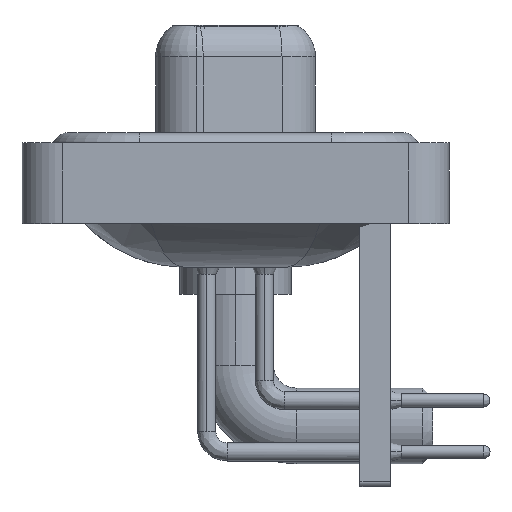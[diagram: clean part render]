
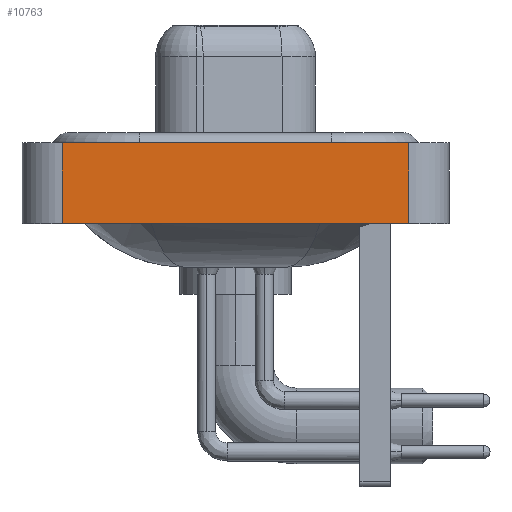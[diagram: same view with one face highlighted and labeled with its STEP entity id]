
A CAD part, left-side view. The second image highlights one B-rep face of the part: STEP entity #10763.
In plain terms, the highlighted planar face has unit normal (-1, 0, 0).
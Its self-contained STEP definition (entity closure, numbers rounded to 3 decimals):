
#282 = CARTESIAN_POINT ( 'NONE',  ( -7.25, -8.55, -3.6 ) ) ;
#705 = VERTEX_POINT ( 'NONE', #17189 ) ;
#1591 = EDGE_CURVE ( 'NONE', #705, #3271, #16674, .T. ) ;
#1983 = EDGE_CURVE ( 'NONE', #16184, #3271, #9719, .T. ) ;
#2035 = VECTOR ( 'NONE', #11398, 1000. ) ;
#2702 = VECTOR ( 'NONE', #7705, 1000. ) ;
#2917 = CARTESIAN_POINT ( 'NONE',  ( -7.25, -8.55, 0.4 ) ) ;
#3153 = ORIENTED_EDGE ( 'NONE', *, *, #8370, .F. ) ;
#3271 = VERTEX_POINT ( 'NONE', #2917 ) ;
#3435 = CARTESIAN_POINT ( 'NONE',  ( -7.25, 8.55, -3.6 ) ) ;
#3968 = DIRECTION ( 'NONE',  ( 0., -1., 0. ) ) ;
#4445 = LINE ( 'NONE', #12413, #2702 ) ;
#5034 = ORIENTED_EDGE ( 'NONE', *, *, #1983, .T. ) ;
#5622 = LINE ( 'NONE', #20192, #10661 ) ;
#5769 = AXIS2_PLACEMENT_3D ( 'NONE', #12751, #14438, #7633 ) ;
#5783 = ORIENTED_EDGE ( 'NONE', *, *, #9924, .T. ) ;
#5931 = DIRECTION ( 'NONE',  ( 0., 0., 1. ) ) ;
#7025 = CARTESIAN_POINT ( 'NONE',  ( -7.25, -8.55, 0.4 ) ) ;
#7633 = DIRECTION ( 'NONE',  ( 0., 0., 1. ) ) ;
#7705 = DIRECTION ( 'NONE',  ( 0., -1., 0. ) ) ;
#8370 = EDGE_CURVE ( 'NONE', #14598, #705, #5622, .T. ) ;
#9719 = LINE ( 'NONE', #282, #2035 ) ;
#9924 = EDGE_CURVE ( 'NONE', #14598, #16184, #4445, .T. ) ;
#10661 = VECTOR ( 'NONE', #5931, 1000. ) ;
#10667 = FACE_OUTER_BOUND ( 'NONE', #15027, .T. ) ;
#10763 = ADVANCED_FACE ( 'NONE', ( #10667 ), #17382, .T. ) ;
#11398 = DIRECTION ( 'NONE',  ( 0., 0., 1. ) ) ;
#12413 = CARTESIAN_POINT ( 'NONE',  ( -7.25, -8.55, -3.6 ) ) ;
#12601 = ORIENTED_EDGE ( 'NONE', *, *, #1591, .F. ) ;
#12751 = CARTESIAN_POINT ( 'NONE',  ( -7.25, -8.55, -3.6 ) ) ;
#14136 = VECTOR ( 'NONE', #3968, 1000. ) ;
#14438 = DIRECTION ( 'NONE',  ( -1., 0., 0. ) ) ;
#14598 = VERTEX_POINT ( 'NONE', #3435 ) ;
#15027 = EDGE_LOOP ( 'NONE', ( #5034, #12601, #3153, #5783 ) ) ;
#16184 = VERTEX_POINT ( 'NONE', #18546 ) ;
#16674 = LINE ( 'NONE', #7025, #14136 ) ;
#17189 = CARTESIAN_POINT ( 'NONE',  ( -7.25, 8.55, 0.4 ) ) ;
#17382 = PLANE ( 'NONE',  #5769 ) ;
#18546 = CARTESIAN_POINT ( 'NONE',  ( -7.25, -8.55, -3.6 ) ) ;
#20192 = CARTESIAN_POINT ( 'NONE',  ( -7.25, 8.55, -3.6 ) ) ;
